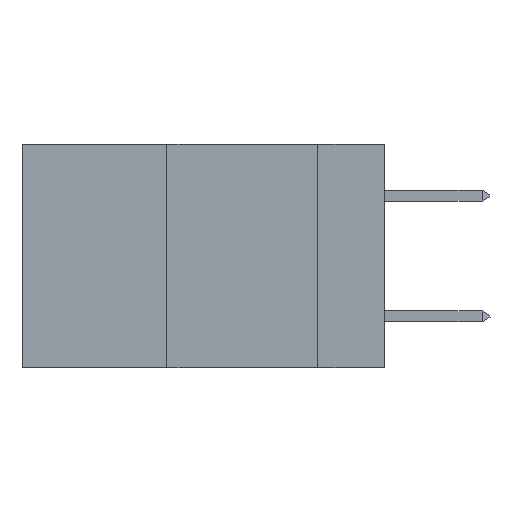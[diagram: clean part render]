
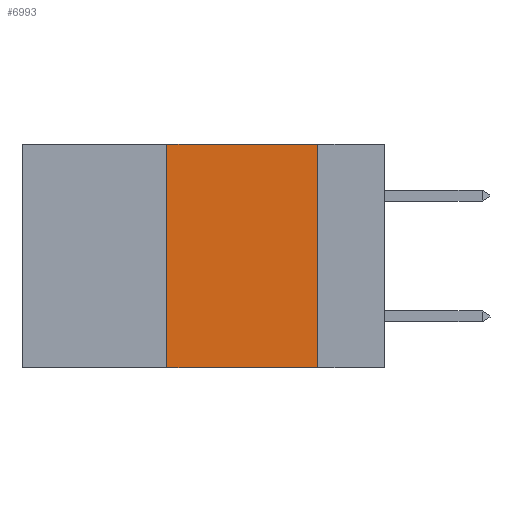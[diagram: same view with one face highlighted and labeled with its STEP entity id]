
A CAD part, left-side view. The second image highlights one B-rep face of the part: STEP entity #6993.
In plain terms, the highlighted planar face has unit normal (-1, 0, 0).
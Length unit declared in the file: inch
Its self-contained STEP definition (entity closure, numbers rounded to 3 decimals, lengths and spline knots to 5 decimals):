
#185 = VERTEX_POINT ( 'NONE', #9093 ) ;
#322 = LINE ( 'NONE', #5378, #3150 ) ;
#656 = FACE_OUTER_BOUND ( 'NONE', #7757, .T. ) ;
#720 = EDGE_CURVE ( 'NONE', #1271, #185, #322, .T. ) ;
#782 = EDGE_CURVE ( 'NONE', #12613, #1928, #8619, .T. ) ;
#862 = EDGE_CURVE ( 'NONE', #12613, #185, #7591, .T. ) ;
#1043 = AXIS2_PLACEMENT_3D ( 'NONE', #13254, #11447, #5283 ) ;
#1074 = CARTESIAN_POINT ( 'NONE',  ( 0., 0.6, -0.37 ) ) ;
#1271 = VERTEX_POINT ( 'NONE', #9780 ) ;
#1928 = VERTEX_POINT ( 'NONE', #11271 ) ;
#2027 = CARTESIAN_POINT ( 'NONE',  ( 0., 0.36, -0.37 ) ) ;
#2229 = ORIENTED_EDGE ( 'NONE', *, *, #720, .F. ) ;
#2785 = CARTESIAN_POINT ( 'NONE',  ( 0., 0.6, 0. ) ) ;
#3150 = VECTOR ( 'NONE', #7680, 39.37008 ) ;
#5283 = DIRECTION ( 'NONE',  ( 0., 0., -1. ) ) ;
#5378 = CARTESIAN_POINT ( 'NONE',  ( 0., 0.11, 0. ) ) ;
#6083 = VECTOR ( 'NONE', #13101, 39.37008 ) ;
#6100 = ORIENTED_EDGE ( 'NONE', *, *, #10761, .F. ) ;
#6301 = ORIENTED_EDGE ( 'NONE', *, *, #782, .F. ) ;
#6993 = ADVANCED_FACE ( 'NONE', ( #656 ), #10518, .F. ) ;
#7128 = ORIENTED_EDGE ( 'NONE', *, *, #862, .T. ) ;
#7591 = LINE ( 'NONE', #1074, #10069 ) ;
#7680 = DIRECTION ( 'NONE',  ( 0., 0., -1. ) ) ;
#7694 = CARTESIAN_POINT ( 'NONE',  ( 0., 0.36, 0. ) ) ;
#7757 = EDGE_LOOP ( 'NONE', ( #2229, #6100, #6301, #7128 ) ) ;
#7995 = DIRECTION ( 'NONE',  ( 0., 0., 1. ) ) ;
#8619 = LINE ( 'NONE', #7694, #13092 ) ;
#9019 = LINE ( 'NONE', #2785, #6083 ) ;
#9078 = DIRECTION ( 'NONE',  ( 0., -1., 0. ) ) ;
#9093 = CARTESIAN_POINT ( 'NONE',  ( 0., 0.11, -0.37 ) ) ;
#9780 = CARTESIAN_POINT ( 'NONE',  ( 0., 0.11, 0. ) ) ;
#10069 = VECTOR ( 'NONE', #9078, 39.37008 ) ;
#10518 = PLANE ( 'NONE',  #1043 ) ;
#10761 = EDGE_CURVE ( 'NONE', #1928, #1271, #9019, .T. ) ;
#11271 = CARTESIAN_POINT ( 'NONE',  ( 0., 0.36, 0. ) ) ;
#11447 = DIRECTION ( 'NONE',  ( 1., 0., 0. ) ) ;
#12613 = VERTEX_POINT ( 'NONE', #2027 ) ;
#13092 = VECTOR ( 'NONE', #7995, 39.37008 ) ;
#13101 = DIRECTION ( 'NONE',  ( 0., -1., 0. ) ) ;
#13254 = CARTESIAN_POINT ( 'NONE',  ( 0., 0.6, 0. ) ) ;
